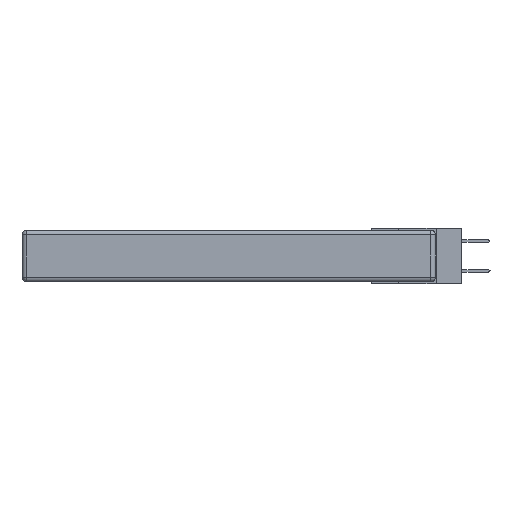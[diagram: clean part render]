
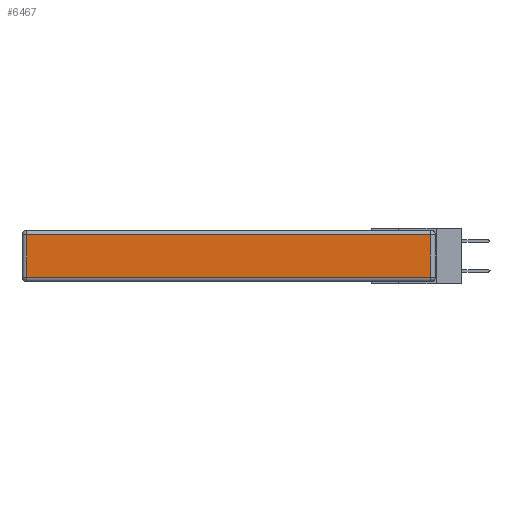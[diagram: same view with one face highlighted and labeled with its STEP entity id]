
A CAD part, left-side view. The second image highlights one B-rep face of the part: STEP entity #6467.
In plain terms, the highlighted planar face has unit normal (-1, 0, 0).
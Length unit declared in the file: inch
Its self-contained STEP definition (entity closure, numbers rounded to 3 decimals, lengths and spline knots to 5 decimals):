
#144 = FACE_OUTER_BOUND ( 'NONE', #4775, .T. ) ;
#250 = CARTESIAN_POINT ( 'NONE',  ( 0., 0., -0.343 ) ) ;
#317 = DIRECTION ( 'NONE',  ( 0., 0., 1. ) ) ;
#1498 = ORIENTED_EDGE ( 'NONE', *, *, #16419, .T. ) ;
#1816 = CARTESIAN_POINT ( 'NONE',  ( 0., 0.03, -0.313 ) ) ;
#2446 = CARTESIAN_POINT ( 'NONE',  ( 0., 2.72, -0.313 ) ) ;
#2500 = ORIENTED_EDGE ( 'NONE', *, *, #19626, .T. ) ;
#2992 = EDGE_CURVE ( 'NONE', #16609, #12658, #11141, .T. ) ;
#4170 = VERTEX_POINT ( 'NONE', #15287 ) ;
#4775 = EDGE_LOOP ( 'NONE', ( #6290, #2500, #8751, #1498 ) ) ;
#4924 = PLANE ( 'NONE',  #12656 ) ;
#6290 = ORIENTED_EDGE ( 'NONE', *, *, #2992, .T. ) ;
#6467 = ADVANCED_FACE ( 'NONE', ( #144 ), #4924, .T. ) ;
#6853 = VECTOR ( 'NONE', #9171, 39.37008 ) ;
#8751 = ORIENTED_EDGE ( 'NONE', *, *, #16831, .T. ) ;
#9171 = DIRECTION ( 'NONE',  ( 0., 1., 0. ) ) ;
#10820 = CARTESIAN_POINT ( 'NONE',  ( 0., 0.03, -0.343 ) ) ;
#11141 = LINE ( 'NONE', #17266, #19874 ) ;
#12591 = CARTESIAN_POINT ( 'NONE',  ( 0., 2.72, -0.343 ) ) ;
#12656 = AXIS2_PLACEMENT_3D ( 'NONE', #250, #14240, #317 ) ;
#12658 = VERTEX_POINT ( 'NONE', #1816 ) ;
#12911 = DIRECTION ( 'NONE',  ( 0., 0., -1. ) ) ;
#13552 = DIRECTION ( 'NONE',  ( 0., 0., 1. ) ) ;
#14101 = LINE ( 'NONE', #10820, #16787 ) ;
#14240 = DIRECTION ( 'NONE',  ( -1., 0., 0. ) ) ;
#14262 = DIRECTION ( 'NONE',  ( 0., -1., 0. ) ) ;
#15074 = LINE ( 'NONE', #12591, #15796 ) ;
#15141 = VERTEX_POINT ( 'NONE', #15283 ) ;
#15283 = CARTESIAN_POINT ( 'NONE',  ( 0., 2.72, -0.03 ) ) ;
#15287 = CARTESIAN_POINT ( 'NONE',  ( 0., 0.03, -0.03 ) ) ;
#15300 = CARTESIAN_POINT ( 'NONE',  ( 0., 2.75, -0.03 ) ) ;
#15796 = VECTOR ( 'NONE', #12911, 39.37008 ) ;
#16419 = EDGE_CURVE ( 'NONE', #15141, #16609, #15074, .T. ) ;
#16609 = VERTEX_POINT ( 'NONE', #2446 ) ;
#16787 = VECTOR ( 'NONE', #13552, 39.37008 ) ;
#16831 = EDGE_CURVE ( 'NONE', #4170, #15141, #18715, .T. ) ;
#17266 = CARTESIAN_POINT ( 'NONE',  ( 0., 0., -0.313 ) ) ;
#18715 = LINE ( 'NONE', #15300, #6853 ) ;
#19626 = EDGE_CURVE ( 'NONE', #12658, #4170, #14101, .T. ) ;
#19874 = VECTOR ( 'NONE', #14262, 39.37008 ) ;
